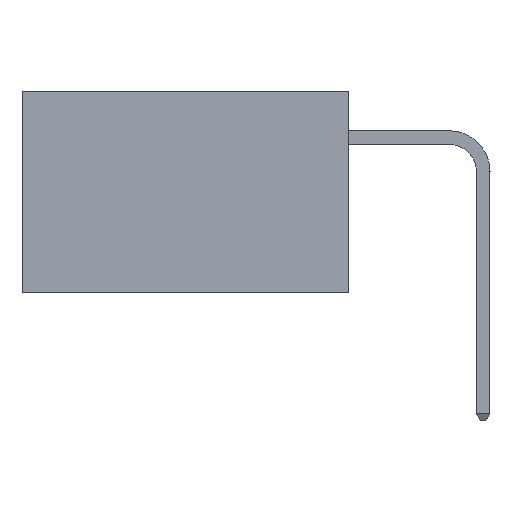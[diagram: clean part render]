
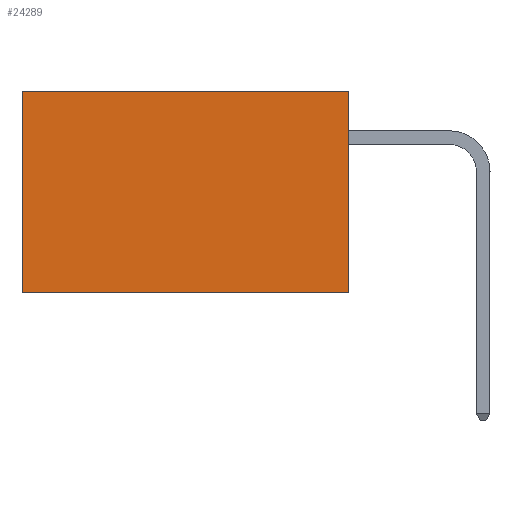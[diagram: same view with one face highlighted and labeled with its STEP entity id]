
A CAD part, left-side view. The second image highlights one B-rep face of the part: STEP entity #24289.
In plain terms, the highlighted planar face has unit normal (-1, 0, 0).
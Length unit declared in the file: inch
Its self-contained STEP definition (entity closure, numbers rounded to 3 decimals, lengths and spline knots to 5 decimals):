
#279 = CARTESIAN_POINT ( 'NONE',  ( 0.2875, 0.6, 0. ) ) ;
#578 = ORIENTED_EDGE ( 'NONE', *, *, #38597, .F. ) ;
#1021 = VERTEX_POINT ( 'NONE', #35831 ) ;
#3435 = DIRECTION ( 'NONE',  ( 0., 0., -1. ) ) ;
#4671 = CARTESIAN_POINT ( 'NONE',  ( 0.2875, 0., 0. ) ) ;
#7197 = VERTEX_POINT ( 'NONE', #28653 ) ;
#7809 = DIRECTION ( 'NONE',  ( 0., 1., 0. ) ) ;
#7860 = VECTOR ( 'NONE', #27847, 39.37008 ) ;
#8291 = CARTESIAN_POINT ( 'NONE',  ( 0.2875, 0.6, 0. ) ) ;
#8821 = LINE ( 'NONE', #24654, #7860 ) ;
#9762 = ORIENTED_EDGE ( 'NONE', *, *, #40168, .T. ) ;
#11934 = EDGE_CURVE ( 'NONE', #1021, #7197, #8821, .T. ) ;
#12574 = LINE ( 'NONE', #279, #18949 ) ;
#14059 = ORIENTED_EDGE ( 'NONE', *, *, #11934, .F. ) ;
#15130 = PLANE ( 'NONE',  #34550 ) ;
#15743 = LINE ( 'NONE', #4671, #31551 ) ;
#15884 = EDGE_LOOP ( 'NONE', ( #9762, #578, #14059, #35186 ) ) ;
#18324 = CARTESIAN_POINT ( 'NONE',  ( 0.2875, 0., 0. ) ) ;
#18949 = VECTOR ( 'NONE', #3435, 39.37008 ) ;
#19550 = VERTEX_POINT ( 'NONE', #8291 ) ;
#21483 = DIRECTION ( 'NONE',  ( 0., 0., -1. ) ) ;
#22538 = VECTOR ( 'NONE', #27391, 39.37008 ) ;
#23170 = FACE_OUTER_BOUND ( 'NONE', #15884, .T. ) ;
#24289 = ADVANCED_FACE ( 'NONE', ( #23170 ), #15130, .F. ) ;
#24515 = LINE ( 'NONE', #36745, #22538 ) ;
#24654 = CARTESIAN_POINT ( 'NONE',  ( 0.2875, 0., 0. ) ) ;
#24708 = EDGE_CURVE ( 'NONE', #1021, #19550, #15743, .T. ) ;
#26592 = VERTEX_POINT ( 'NONE', #40084 ) ;
#27391 = DIRECTION ( 'NONE',  ( 0., 1., 0. ) ) ;
#27847 = DIRECTION ( 'NONE',  ( 0., 0., -1. ) ) ;
#28653 = CARTESIAN_POINT ( 'NONE',  ( 0.2875, 0., -0.37 ) ) ;
#31551 = VECTOR ( 'NONE', #7809, 39.37008 ) ;
#34550 = AXIS2_PLACEMENT_3D ( 'NONE', #18324, #40373, #21483 ) ;
#35186 = ORIENTED_EDGE ( 'NONE', *, *, #24708, .T. ) ;
#35831 = CARTESIAN_POINT ( 'NONE',  ( 0.2875, 0., 0. ) ) ;
#36745 = CARTESIAN_POINT ( 'NONE',  ( 0.2875, 0., -0.37 ) ) ;
#38597 = EDGE_CURVE ( 'NONE', #7197, #26592, #24515, .T. ) ;
#40084 = CARTESIAN_POINT ( 'NONE',  ( 0.2875, 0.6, -0.37 ) ) ;
#40168 = EDGE_CURVE ( 'NONE', #19550, #26592, #12574, .T. ) ;
#40373 = DIRECTION ( 'NONE',  ( 1., 0., 0. ) ) ;
